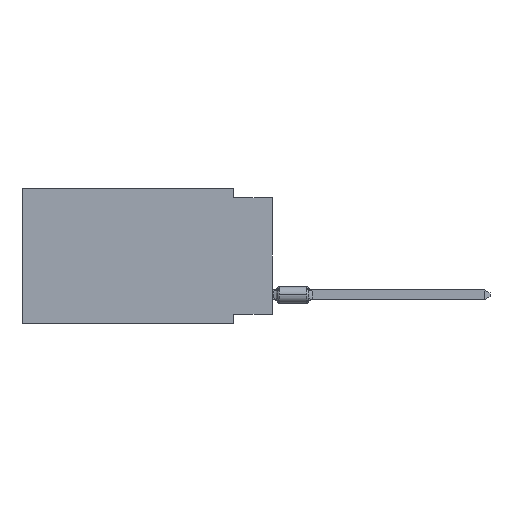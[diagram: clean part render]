
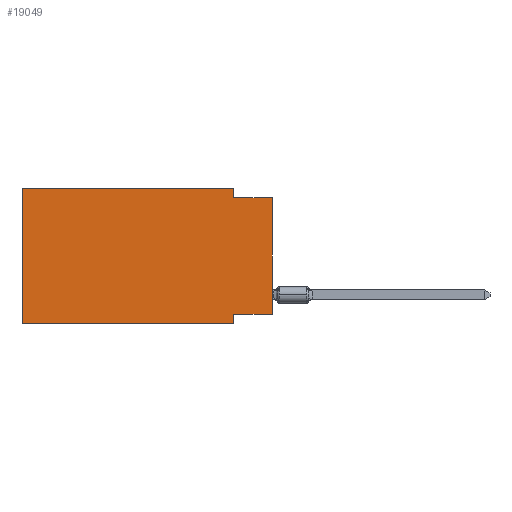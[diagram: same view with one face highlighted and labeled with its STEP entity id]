
A CAD part, left-side view. The second image highlights one B-rep face of the part: STEP entity #19049.
In plain terms, the highlighted planar face has unit normal (-1, 0, 0).
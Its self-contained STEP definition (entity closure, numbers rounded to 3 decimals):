
#39 = DIRECTION ( 'NONE',  ( 0., -1., 0. ) ) ;
#378 = LINE ( 'NONE', #9415, #7952 ) ;
#524 = DIRECTION ( 'NONE',  ( 0., -1., 0. ) ) ;
#665 = EDGE_CURVE ( 'NONE', #6817, #17196, #5096, .T. ) ;
#856 = VECTOR ( 'NONE', #14599, 1000. ) ;
#1028 = VECTOR ( 'NONE', #524, 1000. ) ;
#1155 = VECTOR ( 'NONE', #39, 1000. ) ;
#1577 = DIRECTION ( 'NONE',  ( 0., 0., -1. ) ) ;
#1594 = EDGE_CURVE ( 'NONE', #6071, #17196, #13837, .T. ) ;
#1625 = ORIENTED_EDGE ( 'NONE', *, *, #5305, .F. ) ;
#1975 = DIRECTION ( 'NONE',  ( 1., 0., 0. ) ) ;
#2202 = LINE ( 'NONE', #8556, #856 ) ;
#2808 = LINE ( 'NONE', #18176, #4452 ) ;
#3629 = CARTESIAN_POINT ( 'NONE',  ( 0., 2.54, -8.255 ) ) ;
#3635 = VERTEX_POINT ( 'NONE', #13533 ) ;
#3674 = FACE_OUTER_BOUND ( 'NONE', #6967, .T. ) ;
#4171 = CARTESIAN_POINT ( 'NONE',  ( 0., 2.54, -8.89 ) ) ;
#4284 = DIRECTION ( 'NONE',  ( 0., 1., 0. ) ) ;
#4452 = VECTOR ( 'NONE', #4284, 1000. ) ;
#4493 = VECTOR ( 'NONE', #1577, 1000. ) ;
#4587 = EDGE_CURVE ( 'NONE', #3635, #6355, #378, .T. ) ;
#4752 = LINE ( 'NONE', #15472, #4493 ) ;
#4870 = ORIENTED_EDGE ( 'NONE', *, *, #18740, .F. ) ;
#5096 = LINE ( 'NONE', #15708, #1028 ) ;
#5305 = EDGE_CURVE ( 'NONE', #6071, #11152, #2808, .T. ) ;
#5644 = VERTEX_POINT ( 'NONE', #4171 ) ;
#5911 = EDGE_CURVE ( 'NONE', #12645, #6817, #4752, .T. ) ;
#6071 = VERTEX_POINT ( 'NONE', #13569 ) ;
#6355 = VERTEX_POINT ( 'NONE', #18922 ) ;
#6817 = VERTEX_POINT ( 'NONE', #14233 ) ;
#6967 = EDGE_LOOP ( 'NONE', ( #10572, #16815, #17597, #9016, #17032, #12544, #4870, #1625 ) ) ;
#7952 = VECTOR ( 'NONE', #11003, 1000. ) ;
#8037 = DIRECTION ( 'NONE',  ( 0., 0., -1. ) ) ;
#8113 = CARTESIAN_POINT ( 'NONE',  ( 0., 0., -0.635 ) ) ;
#8556 = CARTESIAN_POINT ( 'NONE',  ( 0., 16.383, 0. ) ) ;
#8889 = LINE ( 'NONE', #15027, #1155 ) ;
#8978 = DIRECTION ( 'NONE',  ( 0., 0., 1. ) ) ;
#9016 = ORIENTED_EDGE ( 'NONE', *, *, #9754, .F. ) ;
#9081 = EDGE_CURVE ( 'NONE', #3635, #5644, #8889, .T. ) ;
#9415 = CARTESIAN_POINT ( 'NONE',  ( 0., 16.383, 0. ) ) ;
#9754 = EDGE_CURVE ( 'NONE', #6355, #12645, #2202, .T. ) ;
#10316 = LINE ( 'NONE', #12017, #15459 ) ;
#10345 = CARTESIAN_POINT ( 'NONE',  ( 0., 2.54, 0. ) ) ;
#10572 = ORIENTED_EDGE ( 'NONE', *, *, #1594, .T. ) ;
#11003 = DIRECTION ( 'NONE',  ( 0., 0., 1. ) ) ;
#11152 = VERTEX_POINT ( 'NONE', #3629 ) ;
#12017 = CARTESIAN_POINT ( 'NONE',  ( 0., 2.54, -8.89 ) ) ;
#12544 = ORIENTED_EDGE ( 'NONE', *, *, #9081, .T. ) ;
#12645 = VERTEX_POINT ( 'NONE', #10345 ) ;
#13113 = DIRECTION ( 'NONE',  ( 0., 0., -1. ) ) ;
#13533 = CARTESIAN_POINT ( 'NONE',  ( 0., 16.383, -8.89 ) ) ;
#13569 = CARTESIAN_POINT ( 'NONE',  ( 0., 0., -8.255 ) ) ;
#13837 = LINE ( 'NONE', #16717, #15951 ) ;
#14233 = CARTESIAN_POINT ( 'NONE',  ( 0., 2.54, -0.635 ) ) ;
#14599 = DIRECTION ( 'NONE',  ( 0., -1., 0. ) ) ;
#15027 = CARTESIAN_POINT ( 'NONE',  ( 0., 16.383, -8.89 ) ) ;
#15459 = VECTOR ( 'NONE', #13113, 1000. ) ;
#15472 = CARTESIAN_POINT ( 'NONE',  ( 0., 2.54, 0. ) ) ;
#15708 = CARTESIAN_POINT ( 'NONE',  ( 0., 0., -0.635 ) ) ;
#15773 = PLANE ( 'NONE',  #19599 ) ;
#15951 = VECTOR ( 'NONE', #8978, 1000. ) ;
#16717 = CARTESIAN_POINT ( 'NONE',  ( 0., 0., 0. ) ) ;
#16815 = ORIENTED_EDGE ( 'NONE', *, *, #665, .F. ) ;
#17032 = ORIENTED_EDGE ( 'NONE', *, *, #4587, .F. ) ;
#17196 = VERTEX_POINT ( 'NONE', #8113 ) ;
#17597 = ORIENTED_EDGE ( 'NONE', *, *, #5911, .F. ) ;
#18176 = CARTESIAN_POINT ( 'NONE',  ( 0., 0., -8.255 ) ) ;
#18740 = EDGE_CURVE ( 'NONE', #11152, #5644, #10316, .T. ) ;
#18922 = CARTESIAN_POINT ( 'NONE',  ( 0., 16.383, 0. ) ) ;
#19049 = ADVANCED_FACE ( 'NONE', ( #3674 ), #15773, .F. ) ;
#19051 = CARTESIAN_POINT ( 'NONE',  ( 0., 16.383, 0. ) ) ;
#19599 = AXIS2_PLACEMENT_3D ( 'NONE', #19051, #1975, #8037 ) ;
